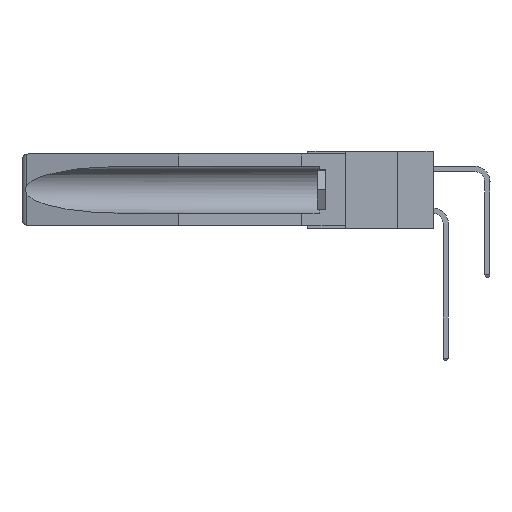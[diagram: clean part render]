
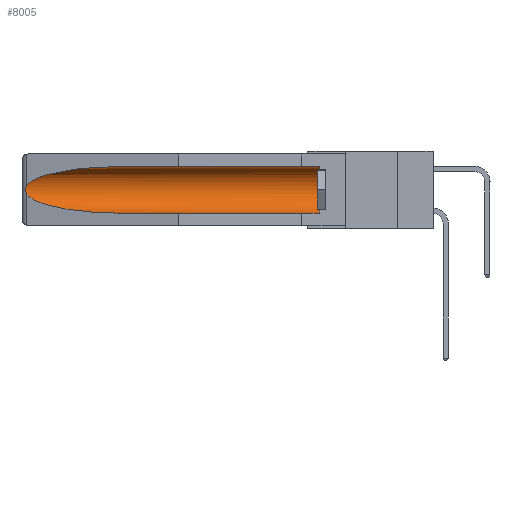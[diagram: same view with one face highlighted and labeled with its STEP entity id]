
A CAD part, left-side view. The second image highlights one B-rep face of the part: STEP entity #8005.
In plain terms, the highlighted cylindrical face has radius 2.857 mm (diameter 5.715 mm), a partial arc.
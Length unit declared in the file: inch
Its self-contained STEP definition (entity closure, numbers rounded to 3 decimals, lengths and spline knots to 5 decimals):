
#109 = CARTESIAN_POINT ( 'NONE',  ( 0.26537, 1.52718, -0.19328 ) ) ;
#182 = CARTESIAN_POINT ( 'NONE',  ( 0.21114, 1.30732, -0.059 ) ) ;
#392 = CARTESIAN_POINT ( 'NONE',  ( 0.155, 0.126, -0.284 ) ) ;
#1543 = CARTESIAN_POINT ( 'NONE',  ( 0.26537, 1.52718, -0.14972 ) ) ;
#1825 = CARTESIAN_POINT ( 'NONE',  ( 0.155, 1.07973, -0.059 ) ) ;
#2225 = VERTEX_POINT ( 'NONE', #12301 ) ;
#2421 = EDGE_CURVE ( 'NONE', #21232, #2225, #15962, .T. ) ;
#2534 = ORIENTED_EDGE ( 'NONE', *, *, #9385, .T. ) ;
#2583 = AXIS2_PLACEMENT_3D ( 'NONE', #12306, #13995, #15732 ) ;
#3243 = CARTESIAN_POINT ( 'NONE',  ( 0.155, -0.30754, -0.284 ) ) ;
#3583 = CARTESIAN_POINT ( 'NONE',  ( 0.155, -0.30754, -0.059 ) ) ;
#3800 = CARTESIAN_POINT ( 'NONE',  ( 0.26537, 1.52718, -0.14972 ) ) ;
#4329 = CARTESIAN_POINT ( 'NONE',  ( 0.155, -0.30754, -0.1715 ) ) ;
#4687 = DIRECTION ( 'NONE',  ( 0., 1., 0. ) ) ;
#5746 = CARTESIAN_POINT ( 'NONE',  ( 0.26537, 1.52718, -0.14972 ) ) ;
#5893 = CARTESIAN_POINT ( 'NONE',  ( 0.2673, 1.5327, -0.16383 ) ) ;
#5989 = CYLINDRICAL_SURFACE ( 'NONE', #20458, 0.1125 ) ;
#7479 = EDGE_LOOP ( 'NONE', ( #19738, #2534, #17511, #8764, #17210, #19990 ) ) ;
#8005 = ADVANCED_FACE ( 'NONE', ( #16603 ), #5989, .F. ) ;
#8187 = VERTEX_POINT ( 'NONE', #10451 ) ;
#8265 = VERTEX_POINT ( 'NONE', #392 ) ;
#8302 = DIRECTION ( 'NONE',  ( 0., 0., 1. ) ) ;
#8764 = ORIENTED_EDGE ( 'NONE', *, *, #21735, .F. ) ;
#9144 = B_SPLINE_CURVE_WITH_KNOTS ( 'NONE', 3,
 ( #5746, #19332, #20916, #5893, #9299, #10874, #15753, #9222, #21149, #10940 ),
 .UNSPECIFIED., .F., .F.,
 ( 4, 2, 2, 2, 4 ),
 ( 0., 0.00029, 0.00058, 0.00087, 0.00117 ),
 .UNSPECIFIED. ) ;
#9222 = CARTESIAN_POINT ( 'NONE',  ( 0.26655, 1.53094, -0.18657 ) ) ;
#9299 = CARTESIAN_POINT ( 'NONE',  ( 0.2675, 1.53308, -0.16763 ) ) ;
#9385 = EDGE_CURVE ( 'NONE', #9721, #21232, #9144, .T. ) ;
#9589 = DIRECTION ( 'NONE',  ( 0., 1., 0. ) ) ;
#9721 = VERTEX_POINT ( 'NONE', #1543 ) ;
#10451 = CARTESIAN_POINT ( 'NONE',  ( 0.155, 0.126, -0.059 ) ) ;
#10874 = CARTESIAN_POINT ( 'NONE',  ( 0.2675, 1.53308, -0.17534 ) ) ;
#10940 = CARTESIAN_POINT ( 'NONE',  ( 0.26537, 1.52718, -0.19328 ) ) ;
#11473 = EDGE_CURVE ( 'NONE', #8187, #21797, #15173, .T. ) ;
#12301 = CARTESIAN_POINT ( 'NONE',  ( 0.155, 1.07973, -0.284 ) ) ;
#12306 = CARTESIAN_POINT ( 'NONE',  ( 0.155, 0.126, -0.1715 ) ) ;
#12798 = CARTESIAN_POINT ( 'NONE',  ( 0.155, 1.07973, -0.284 ) ) ;
#13064 = EDGE_CURVE ( 'NONE', #8265, #8187, #13364, .T. ) ;
#13364 = CIRCLE ( 'NONE', #2583, 0.1125 ) ;
#13995 = DIRECTION ( 'NONE',  ( 0., -1., 0. ) ) ;
#14362 = CARTESIAN_POINT ( 'NONE',  ( 0.26537, 1.52718, -0.19328 ) ) ;
#14444 = CARTESIAN_POINT ( 'NONE',  ( 0.25451, 1.48313, -0.24835 ) ) ;
#15173 = LINE ( 'NONE', #3583, #19461 ) ;
#15258 = CARTESIAN_POINT ( 'NONE',  ( 0.155, 1.07973, -0.059 ) ) ;
#15368 = DIRECTION ( 'NONE',  ( 0., 1., 0. ) ) ;
#15674 =( BOUNDED_CURVE ( )  B_SPLINE_CURVE ( 3, ( #1825, #182, #20514, #3800 ),
 .UNSPECIFIED., .F., .F. ) 
 B_SPLINE_CURVE_WITH_KNOTS ( ( 4, 4 ),
 ( 4.71239, 6.08839 ),
 .UNSPECIFIED. ) 
 CURVE ( )  GEOMETRIC_REPRESENTATION_ITEM ( )  RATIONAL_B_SPLINE_CURVE ( ( 1., 0.848, 0.848, 1. ) ) 
 REPRESENTATION_ITEM ( '' )  );
#15732 = DIRECTION ( 'NONE',  ( 0., 0., 1. ) ) ;
#15753 = CARTESIAN_POINT ( 'NONE',  ( 0.2673, 1.53269, -0.17917 ) ) ;
#15936 = LINE ( 'NONE', #3243, #18090 ) ;
#15962 =( BOUNDED_CURVE ( )  B_SPLINE_CURVE ( 3, ( #14362, #14444, #19522, #12798 ),
 .UNSPECIFIED., .F., .F. ) 
 B_SPLINE_CURVE_WITH_KNOTS ( ( 4, 4 ),
 ( 0.1948, 1.5708 ),
 .UNSPECIFIED. ) 
 CURVE ( )  GEOMETRIC_REPRESENTATION_ITEM ( )  RATIONAL_B_SPLINE_CURVE ( ( 1., 0.848, 0.848, 1. ) ) 
 REPRESENTATION_ITEM ( '' )  );
#16603 = FACE_OUTER_BOUND ( 'NONE', #7479, .T. ) ;
#17210 = ORIENTED_EDGE ( 'NONE', *, *, #13064, .T. ) ;
#17511 = ORIENTED_EDGE ( 'NONE', *, *, #2421, .T. ) ;
#18090 = VECTOR ( 'NONE', #4687, 39.37008 ) ;
#18298 = EDGE_CURVE ( 'NONE', #21797, #9721, #15674, .T. ) ;
#19332 = CARTESIAN_POINT ( 'NONE',  ( 0.26597, 1.52961, -0.15275 ) ) ;
#19461 = VECTOR ( 'NONE', #15368, 39.37008 ) ;
#19522 = CARTESIAN_POINT ( 'NONE',  ( 0.21114, 1.30732, -0.284 ) ) ;
#19738 = ORIENTED_EDGE ( 'NONE', *, *, #18298, .T. ) ;
#19990 = ORIENTED_EDGE ( 'NONE', *, *, #11473, .T. ) ;
#20458 = AXIS2_PLACEMENT_3D ( 'NONE', #4329, #9589, #8302 ) ;
#20514 = CARTESIAN_POINT ( 'NONE',  ( 0.25451, 1.48313, -0.09465 ) ) ;
#20916 = CARTESIAN_POINT ( 'NONE',  ( 0.26654, 1.53092, -0.15636 ) ) ;
#21149 = CARTESIAN_POINT ( 'NONE',  ( 0.26597, 1.5296, -0.19026 ) ) ;
#21232 = VERTEX_POINT ( 'NONE', #109 ) ;
#21735 = EDGE_CURVE ( 'NONE', #8265, #2225, #15936, .T. ) ;
#21797 = VERTEX_POINT ( 'NONE', #15258 ) ;
